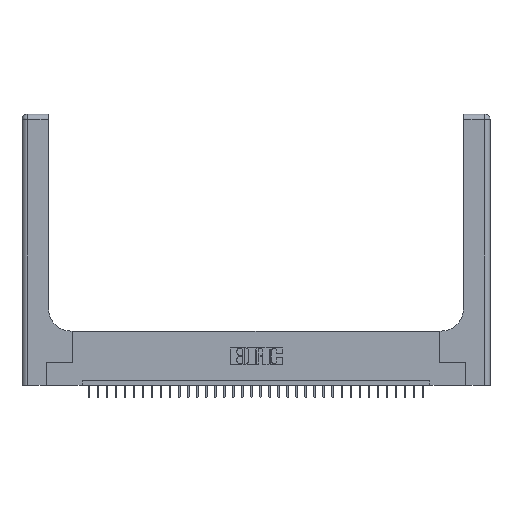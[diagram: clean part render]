
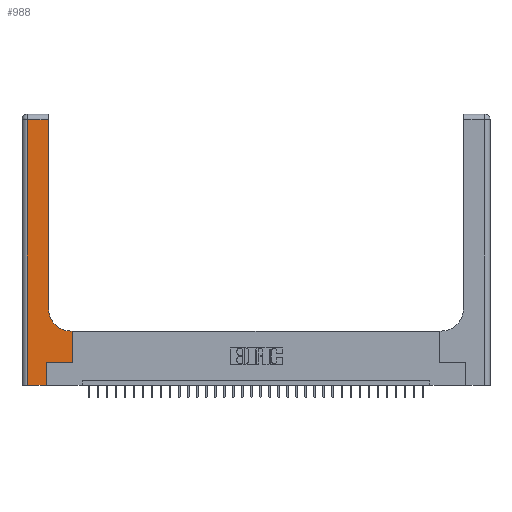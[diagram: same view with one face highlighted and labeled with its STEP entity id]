
A CAD part, top view. The second image highlights one B-rep face of the part: STEP entity #988.
In plain terms, the highlighted planar face has unit normal (0, 0, 1).
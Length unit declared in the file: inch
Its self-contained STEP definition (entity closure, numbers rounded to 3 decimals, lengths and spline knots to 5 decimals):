
#830 = DIRECTION ( 'NONE',  ( -1., 0., 0. ) ) ;
#988 = ADVANCED_FACE ( 'NONE', ( #32828 ), #27597, .F. ) ;
#2321 = VERTEX_POINT ( 'NONE', #4286 ) ;
#2399 = CARTESIAN_POINT ( 'NONE',  ( 0.06, 0., 0.37 ) ) ;
#3614 = LINE ( 'NONE', #11614, #19319 ) ;
#3839 = CARTESIAN_POINT ( 'NONE',  ( 0.5415, 0.6, 0.37 ) ) ;
#4286 = CARTESIAN_POINT ( 'NONE',  ( 0.2915, 2.94, 0.37 ) ) ;
#4744 = ORIENTED_EDGE ( 'NONE', *, *, #26701, .T. ) ;
#4994 = CARTESIAN_POINT ( 'NONE',  ( 0., 2.94, 0.37 ) ) ;
#5219 = VERTEX_POINT ( 'NONE', #12133 ) ;
#5336 = ORIENTED_EDGE ( 'NONE', *, *, #11013, .T. ) ;
#5600 = EDGE_CURVE ( 'NONE', #17125, #25082, #20062, .T. ) ;
#5880 = LINE ( 'NONE', #11092, #5909 ) ;
#5909 = VECTOR ( 'NONE', #21698, 39.37008 ) ;
#5958 = VERTEX_POINT ( 'NONE', #3839 ) ;
#6395 = CARTESIAN_POINT ( 'NONE',  ( 0.06, 3., 0.37 ) ) ;
#6561 = VECTOR ( 'NONE', #15311, 39.37008 ) ;
#6590 = DIRECTION ( 'NONE',  ( 0., 1., 0. ) ) ;
#7182 = VERTEX_POINT ( 'NONE', #33772 ) ;
#7564 = DIRECTION ( 'NONE',  ( 0., 0., -1. ) ) ;
#7684 = CIRCLE ( 'NONE', #12129, 0.25 ) ;
#7985 = EDGE_CURVE ( 'NONE', #7182, #5958, #3614, .T. ) ;
#8591 = ORIENTED_EDGE ( 'NONE', *, *, #7985, .T. ) ;
#9158 = VECTOR ( 'NONE', #6590, 39.37008 ) ;
#9546 = LINE ( 'NONE', #25697, #9158 ) ;
#10027 = ORIENTED_EDGE ( 'NONE', *, *, #12548, .T. ) ;
#10067 = ORIENTED_EDGE ( 'NONE', *, *, #25177, .T. ) ;
#10085 = CARTESIAN_POINT ( 'NONE',  ( 0.2915, 3., 0.37 ) ) ;
#11013 = EDGE_CURVE ( 'NONE', #5958, #24098, #7684, .T. ) ;
#11092 = CARTESIAN_POINT ( 'NONE',  ( 0.269, 0., 0.37 ) ) ;
#11160 = VERTEX_POINT ( 'NONE', #29653 ) ;
#11614 = CARTESIAN_POINT ( 'NONE',  ( 0.2915, 0.6, 0.37 ) ) ;
#12129 = AXIS2_PLACEMENT_3D ( 'NONE', #31216, #7564, #23552 ) ;
#12133 = CARTESIAN_POINT ( 'NONE',  ( 0.5585, 0.25, 0.37 ) ) ;
#12428 = CARTESIAN_POINT ( 'NONE',  ( 0.269, 0.25, 0.37 ) ) ;
#12548 = EDGE_CURVE ( 'NONE', #11160, #5219, #30074, .T. ) ;
#12984 = DIRECTION ( 'NONE',  ( -1., 0., 0. ) ) ;
#13748 = EDGE_CURVE ( 'NONE', #2321, #26244, #23418, .T. ) ;
#13871 = DIRECTION ( 'NONE',  ( 0., -1., 0. ) ) ;
#13930 = VECTOR ( 'NONE', #13871, 39.37008 ) ;
#14073 = CARTESIAN_POINT ( 'NONE',  ( 0.269, 0., 0.37 ) ) ;
#14385 = LINE ( 'NONE', #6395, #13930 ) ;
#15311 = DIRECTION ( 'NONE',  ( 0., 1., 0. ) ) ;
#15773 = EDGE_CURVE ( 'NONE', #24098, #2321, #29235, .T. ) ;
#16421 = EDGE_LOOP ( 'NONE', ( #30565, #33460, #33639, #32453, #4744, #10027, #10067, #8591, #5336 ) ) ;
#16643 = DIRECTION ( 'NONE',  ( -1., 0., 0. ) ) ;
#17125 = VERTEX_POINT ( 'NONE', #2399 ) ;
#18748 = EDGE_CURVE ( 'NONE', #26244, #17125, #14385, .T. ) ;
#19319 = VECTOR ( 'NONE', #830, 39.37008 ) ;
#20062 = LINE ( 'NONE', #25425, #29214 ) ;
#20229 = DIRECTION ( 'NONE',  ( 1., 0., 0. ) ) ;
#21698 = DIRECTION ( 'NONE',  ( 0., 1., 0. ) ) ;
#22178 = VECTOR ( 'NONE', #12984, 39.37008 ) ;
#22226 = DIRECTION ( 'NONE',  ( 1., 0., 0. ) ) ;
#23418 = LINE ( 'NONE', #4994, #22178 ) ;
#23552 = DIRECTION ( 'NONE',  ( 1., 0., 0. ) ) ;
#24098 = VERTEX_POINT ( 'NONE', #32128 ) ;
#25082 = VERTEX_POINT ( 'NONE', #14073 ) ;
#25177 = EDGE_CURVE ( 'NONE', #5219, #7182, #9546, .T. ) ;
#25425 = CARTESIAN_POINT ( 'NONE',  ( 0., 0., 0.37 ) ) ;
#25697 = CARTESIAN_POINT ( 'NONE',  ( 0.5585, 0.25, 0.37 ) ) ;
#26244 = VERTEX_POINT ( 'NONE', #29106 ) ;
#26701 = EDGE_CURVE ( 'NONE', #25082, #11160, #5880, .T. ) ;
#27597 = PLANE ( 'NONE',  #27939 ) ;
#27939 = AXIS2_PLACEMENT_3D ( 'NONE', #32306, #30049, #16643 ) ;
#29106 = CARTESIAN_POINT ( 'NONE',  ( 0.06, 2.94, 0.37 ) ) ;
#29214 = VECTOR ( 'NONE', #20229, 39.37008 ) ;
#29235 = LINE ( 'NONE', #10085, #6561 ) ;
#29653 = CARTESIAN_POINT ( 'NONE',  ( 0.269, 0.25, 0.37 ) ) ;
#30049 = DIRECTION ( 'NONE',  ( 0., 0., -1. ) ) ;
#30074 = LINE ( 'NONE', #12428, #33166 ) ;
#30565 = ORIENTED_EDGE ( 'NONE', *, *, #15773, .T. ) ;
#31216 = CARTESIAN_POINT ( 'NONE',  ( 0.5415, 0.85, 0.37 ) ) ;
#32128 = CARTESIAN_POINT ( 'NONE',  ( 0.2915, 0.85, 0.37 ) ) ;
#32306 = CARTESIAN_POINT ( 'NONE',  ( 0., 3., 0.37 ) ) ;
#32453 = ORIENTED_EDGE ( 'NONE', *, *, #5600, .T. ) ;
#32828 = FACE_OUTER_BOUND ( 'NONE', #16421, .T. ) ;
#33166 = VECTOR ( 'NONE', #22226, 39.37008 ) ;
#33460 = ORIENTED_EDGE ( 'NONE', *, *, #13748, .T. ) ;
#33639 = ORIENTED_EDGE ( 'NONE', *, *, #18748, .T. ) ;
#33772 = CARTESIAN_POINT ( 'NONE',  ( 0.5585, 0.6, 0.37 ) ) ;
